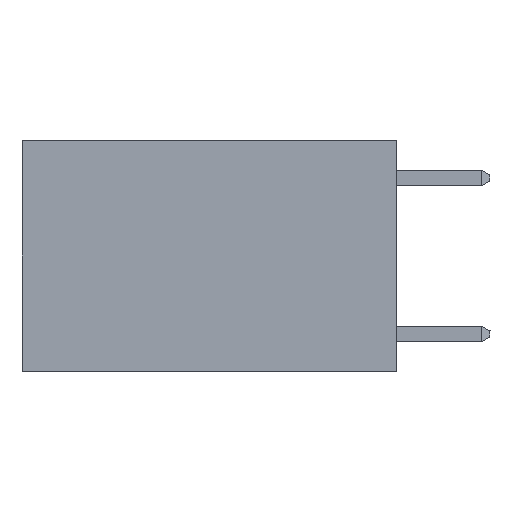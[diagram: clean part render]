
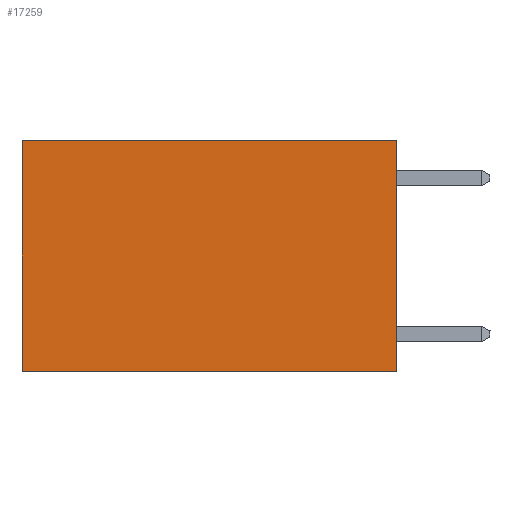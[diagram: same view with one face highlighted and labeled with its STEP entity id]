
A CAD part, left-side view. The second image highlights one B-rep face of the part: STEP entity #17259.
In plain terms, the highlighted planar face has unit normal (-1, 0, 0).
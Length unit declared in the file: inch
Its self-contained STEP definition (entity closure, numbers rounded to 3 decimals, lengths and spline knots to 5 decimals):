
#1541 = AXIS2_PLACEMENT_3D ( 'NONE', #26587, #13178, #28605 ) ;
#1684 = CARTESIAN_POINT ( 'NONE',  ( 0.2625, 0., -0.37 ) ) ;
#1693 = EDGE_CURVE ( 'NONE', #23289, #4356, #17551, .T. ) ;
#3941 = DIRECTION ( 'NONE',  ( 0., 1., 0. ) ) ;
#4356 = VERTEX_POINT ( 'NONE', #18672 ) ;
#5792 = DIRECTION ( 'NONE',  ( 0., 0., -1. ) ) ;
#6328 = ORIENTED_EDGE ( 'NONE', *, *, #10680, .F. ) ;
#7187 = DIRECTION ( 'NONE',  ( 0., 0., -1. ) ) ;
#7204 = VERTEX_POINT ( 'NONE', #10588 ) ;
#7504 = EDGE_LOOP ( 'NONE', ( #27977, #6328, #11009, #12636 ) ) ;
#8771 = LINE ( 'NONE', #23657, #14049 ) ;
#9335 = CARTESIAN_POINT ( 'NONE',  ( 0.2625, 0.6, 0. ) ) ;
#10588 = CARTESIAN_POINT ( 'NONE',  ( 0.2625, 0.6, -0.37 ) ) ;
#10680 = EDGE_CURVE ( 'NONE', #11593, #7204, #16178, .T. ) ;
#11009 = ORIENTED_EDGE ( 'NONE', *, *, #16538, .F. ) ;
#11593 = VERTEX_POINT ( 'NONE', #27936 ) ;
#11898 = CARTESIAN_POINT ( 'NONE',  ( 0.2625, 0., 0. ) ) ;
#12636 = ORIENTED_EDGE ( 'NONE', *, *, #1693, .T. ) ;
#13091 = PLANE ( 'NONE',  #1541 ) ;
#13178 = DIRECTION ( 'NONE',  ( 1., 0., 0. ) ) ;
#14049 = VECTOR ( 'NONE', #5792, 39.37008 ) ;
#16178 = LINE ( 'NONE', #1684, #27245 ) ;
#16538 = EDGE_CURVE ( 'NONE', #23289, #11593, #8771, .T. ) ;
#16554 = LINE ( 'NONE', #9335, #21816 ) ;
#17259 = ADVANCED_FACE ( 'NONE', ( #24554 ), #13091, .F. ) ;
#17551 = LINE ( 'NONE', #11898, #17975 ) ;
#17975 = VECTOR ( 'NONE', #27435, 39.37008 ) ;
#18672 = CARTESIAN_POINT ( 'NONE',  ( 0.2625, 0.6, 0. ) ) ;
#19122 = CARTESIAN_POINT ( 'NONE',  ( 0.2625, 0., 0. ) ) ;
#20139 = EDGE_CURVE ( 'NONE', #4356, #7204, #16554, .T. ) ;
#21816 = VECTOR ( 'NONE', #7187, 39.37008 ) ;
#23289 = VERTEX_POINT ( 'NONE', #19122 ) ;
#23657 = CARTESIAN_POINT ( 'NONE',  ( 0.2625, 0., 0. ) ) ;
#24554 = FACE_OUTER_BOUND ( 'NONE', #7504, .T. ) ;
#26587 = CARTESIAN_POINT ( 'NONE',  ( 0.2625, 0., 0. ) ) ;
#27245 = VECTOR ( 'NONE', #3941, 39.37008 ) ;
#27435 = DIRECTION ( 'NONE',  ( 0., 1., 0. ) ) ;
#27936 = CARTESIAN_POINT ( 'NONE',  ( 0.2625, 0., -0.37 ) ) ;
#27977 = ORIENTED_EDGE ( 'NONE', *, *, #20139, .T. ) ;
#28605 = DIRECTION ( 'NONE',  ( 0., 0., -1. ) ) ;
